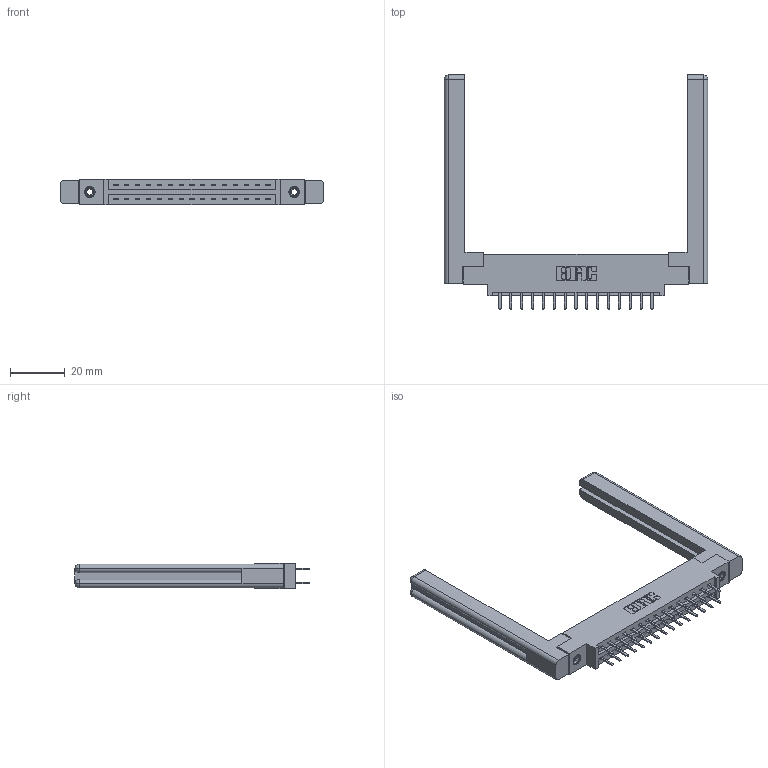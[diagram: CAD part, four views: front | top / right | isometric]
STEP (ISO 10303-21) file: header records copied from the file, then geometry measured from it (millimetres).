
FILE_DESCRIPTION (( 'STEP AP203' ), '1' );
FILE_NAME ('387-030-520-858.STEP', '2019-10-16T23:36:09', ( '' ), ( '' ), 'SwSTEP 2.0', 'SolidWorks 2016', '' );
FILE_SCHEMA (( 'CONFIG_CONTROL_DESIGN' ));
Length unit declared in the file: inch
Products named in the file (5): 307-220-058; 387-030-520-858; 345-250-001_345-250-001-102; 345-292-001_345-293-120; 337 Part_0.170 Offset - 0.156 Dia-TI
Assembly tree (35 placements, depth 2):
  387-030-520-858
    337 Part_0.170 Offset - 0.156 Dia-TI
    345-292-001_345-293-120  x30
    345-250-001_345-250-001-102  x2
    307-220-058  x2
Bounding box: 96.06 x 85.43 x 9.4 mm (x, y, z)
Volume: 16776.1 mm3; surface area: 15745.7 mm2
Topology: 35 solids, 35 shells, 2000 faces, 5747 edges, 3738 vertices
Faces by surface type: plane 1358, cylinder 618, cone 12, torus 12
Entity records: 18002 total; most frequent: CARTESIAN_POINT 3077, ORIENTED_EDGE 2940, DIRECTION 2670, EDGE_CURVE 1470, VECTOR 1290, LINE 1290, VERTEX_POINT 970, AXIS2_PLACEMENT_3D 690
